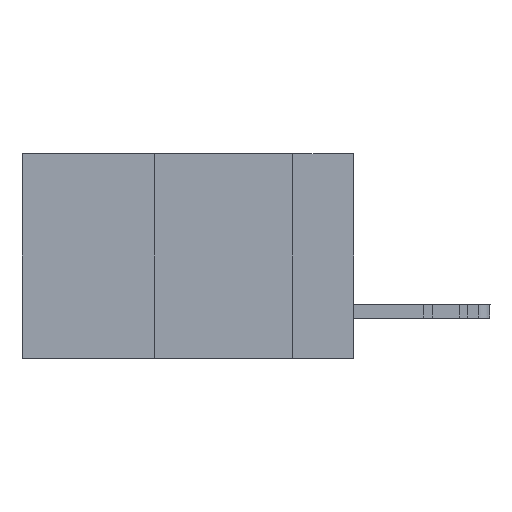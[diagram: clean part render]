
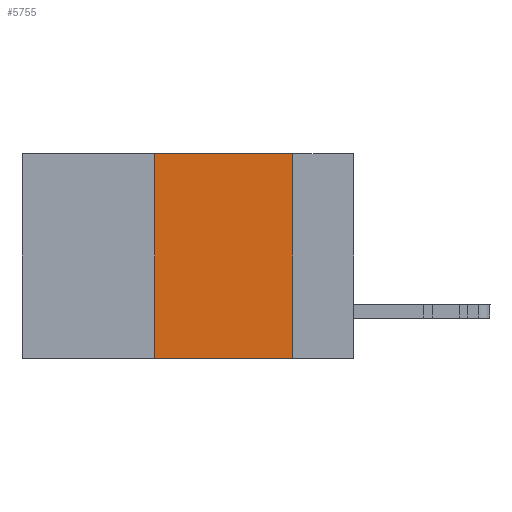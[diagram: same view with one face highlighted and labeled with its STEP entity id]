
A CAD part, left-side view. The second image highlights one B-rep face of the part: STEP entity #5755.
In plain terms, the highlighted planar face has unit normal (-1, 0, 0).
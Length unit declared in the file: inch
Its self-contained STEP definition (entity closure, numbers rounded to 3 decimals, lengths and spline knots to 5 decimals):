
#2464 = ORIENTED_EDGE ( 'NONE', *, *, #31465, .F. ) ;
#4584 = ORIENTED_EDGE ( 'NONE', *, *, #33066, .F. ) ;
#5755 = ADVANCED_FACE ( 'NONE', ( #28952 ), #28720, .F. ) ;
#5882 = DIRECTION ( 'NONE',  ( 0., -1., 0. ) ) ;
#6379 = CARTESIAN_POINT ( 'NONE',  ( 0., 0.11, 0. ) ) ;
#8722 = CARTESIAN_POINT ( 'NONE',  ( 0., 0.36, 0. ) ) ;
#10871 = LINE ( 'NONE', #11331, #15047 ) ;
#11331 = CARTESIAN_POINT ( 'NONE',  ( 0., 0.6, -0.37 ) ) ;
#12361 = VECTOR ( 'NONE', #33436, 39.37008 ) ;
#13590 = LINE ( 'NONE', #6379, #29673 ) ;
#14577 = DIRECTION ( 'NONE',  ( 0., -1., 0. ) ) ;
#15047 = VECTOR ( 'NONE', #14577, 39.37008 ) ;
#15659 = VERTEX_POINT ( 'NONE', #40409 ) ;
#16550 = CARTESIAN_POINT ( 'NONE',  ( 0., 0.6, 0. ) ) ;
#20441 = VERTEX_POINT ( 'NONE', #26345 ) ;
#21756 = CARTESIAN_POINT ( 'NONE',  ( 0., 0.6, 0. ) ) ;
#23493 = LINE ( 'NONE', #16550, #28312 ) ;
#23651 = CARTESIAN_POINT ( 'NONE',  ( 0., 0.36, 0. ) ) ;
#24313 = VERTEX_POINT ( 'NONE', #33599 ) ;
#25156 = EDGE_CURVE ( 'NONE', #24313, #39032, #37831, .T. ) ;
#26345 = CARTESIAN_POINT ( 'NONE',  ( 0., 0.11, 0. ) ) ;
#27224 = EDGE_LOOP ( 'NONE', ( #2464, #4584, #41623, #33152 ) ) ;
#27740 = DIRECTION ( 'NONE',  ( 0., 0., -1. ) ) ;
#28312 = VECTOR ( 'NONE', #5882, 39.37008 ) ;
#28720 = PLANE ( 'NONE',  #39210 ) ;
#28952 = FACE_OUTER_BOUND ( 'NONE', #27224, .T. ) ;
#29673 = VECTOR ( 'NONE', #27740, 39.37008 ) ;
#31465 = EDGE_CURVE ( 'NONE', #20441, #15659, #13590, .T. ) ;
#32891 = DIRECTION ( 'NONE',  ( 0., 0., -1. ) ) ;
#33066 = EDGE_CURVE ( 'NONE', #39032, #20441, #23493, .T. ) ;
#33152 = ORIENTED_EDGE ( 'NONE', *, *, #44099, .T. ) ;
#33436 = DIRECTION ( 'NONE',  ( 0., 0., 1. ) ) ;
#33599 = CARTESIAN_POINT ( 'NONE',  ( 0., 0.36, -0.37 ) ) ;
#37831 = LINE ( 'NONE', #23651, #12361 ) ;
#39032 = VERTEX_POINT ( 'NONE', #8722 ) ;
#39210 = AXIS2_PLACEMENT_3D ( 'NONE', #21756, #42639, #32891 ) ;
#40409 = CARTESIAN_POINT ( 'NONE',  ( 0., 0.11, -0.37 ) ) ;
#41623 = ORIENTED_EDGE ( 'NONE', *, *, #25156, .F. ) ;
#42639 = DIRECTION ( 'NONE',  ( 1., 0., 0. ) ) ;
#44099 = EDGE_CURVE ( 'NONE', #24313, #15659, #10871, .T. ) ;
